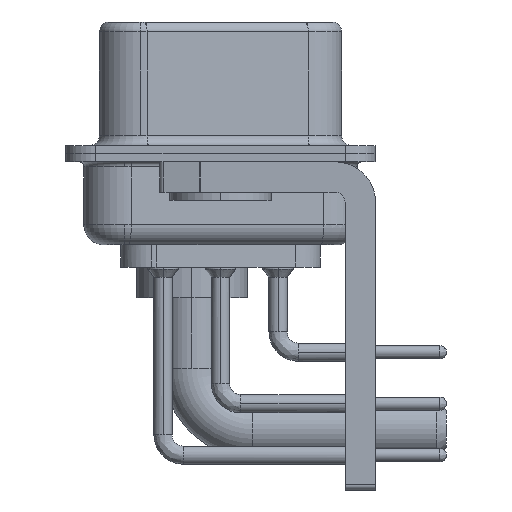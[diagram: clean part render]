
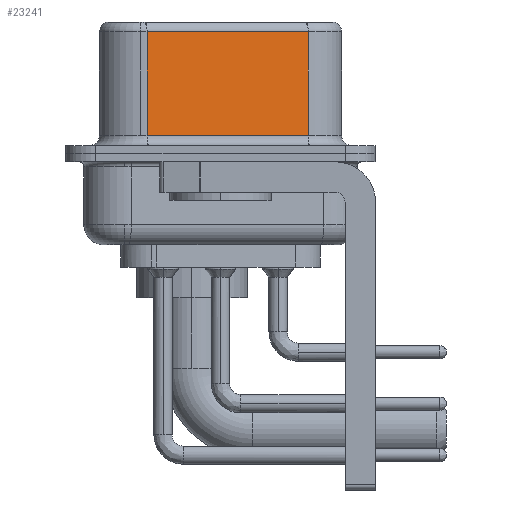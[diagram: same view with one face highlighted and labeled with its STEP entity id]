
A CAD part, left-side view. The second image highlights one B-rep face of the part: STEP entity #23241.
In plain terms, the highlighted planar face has unit normal (-0.985, -0.174, 0).
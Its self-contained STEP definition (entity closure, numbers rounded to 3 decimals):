
#31 = LINE ( 'NONE', #31865, #17573 ) ;
#104 = ORIENTED_EDGE ( 'NONE', *, *, #11338, .T. ) ;
#115 = CARTESIAN_POINT ( 'NONE',  ( 3.73, 3.628, 6.52 ) ) ;
#1654 = CARTESIAN_POINT ( 'NONE',  ( 5.132, -4.322, 6.02 ) ) ;
#2348 = DIRECTION ( 'NONE',  ( 0.985, 0.174, 0. ) ) ;
#4898 = AXIS2_PLACEMENT_3D ( 'NONE', #11787, #2348, #25856 ) ;
#5734 = EDGE_CURVE ( 'NONE', #5994, #14190, #31, .T. ) ;
#5755 = LINE ( 'NONE', #26366, #19918 ) ;
#5922 = DIRECTION ( 'NONE',  ( 0., 0., -1. ) ) ;
#5994 = VERTEX_POINT ( 'NONE', #1654 ) ;
#7140 = VERTEX_POINT ( 'NONE', #18262 ) ;
#9394 = CARTESIAN_POINT ( 'NONE',  ( 5.132, -4.322, 0.9 ) ) ;
#9592 = VECTOR ( 'NONE', #5922, 1000. ) ;
#10969 = DIRECTION ( 'NONE',  ( 0.174, -0.985, 0. ) ) ;
#11338 = EDGE_CURVE ( 'NONE', #7140, #14190, #5755, .T. ) ;
#11705 = LINE ( 'NONE', #115, #9592 ) ;
#11787 = CARTESIAN_POINT ( 'NONE',  ( 5.132, -4.322, 6.52 ) ) ;
#12642 = VECTOR ( 'NONE', #26289, 1000. ) ;
#12917 = EDGE_CURVE ( 'NONE', #5994, #19190, #13971, .T. ) ;
#13510 = CARTESIAN_POINT ( 'NONE',  ( 3.73, 3.628, 6.02 ) ) ;
#13971 = LINE ( 'NONE', #17236, #12642 ) ;
#14190 = VERTEX_POINT ( 'NONE', #9394 ) ;
#14327 = DIRECTION ( 'NONE',  ( 0., 0., -1. ) ) ;
#14500 = ORIENTED_EDGE ( 'NONE', *, *, #31309, .T. ) ;
#17236 = CARTESIAN_POINT ( 'NONE',  ( 5.132, -4.322, 6.02 ) ) ;
#17573 = VECTOR ( 'NONE', #14327, 1000. ) ;
#18262 = CARTESIAN_POINT ( 'NONE',  ( 3.73, 3.628, 0.9 ) ) ;
#19190 = VERTEX_POINT ( 'NONE', #13510 ) ;
#19918 = VECTOR ( 'NONE', #10969, 1000. ) ;
#23241 = ADVANCED_FACE ( 'NONE', ( #28754 ), #26051, .F. ) ;
#25856 = DIRECTION ( 'NONE',  ( -0.174, 0.985, 0. ) ) ;
#26051 = PLANE ( 'NONE',  #4898 ) ;
#26289 = DIRECTION ( 'NONE',  ( -0.174, 0.985, 0. ) ) ;
#26366 = CARTESIAN_POINT ( 'NONE',  ( 5.132, -4.322, 0.9 ) ) ;
#26873 = ORIENTED_EDGE ( 'NONE', *, *, #5734, .F. ) ;
#27369 = EDGE_LOOP ( 'NONE', ( #26873, #27593, #14500, #104 ) ) ;
#27593 = ORIENTED_EDGE ( 'NONE', *, *, #12917, .T. ) ;
#28754 = FACE_OUTER_BOUND ( 'NONE', #27369, .T. ) ;
#31309 = EDGE_CURVE ( 'NONE', #19190, #7140, #11705, .T. ) ;
#31865 = CARTESIAN_POINT ( 'NONE',  ( 5.132, -4.322, 6.52 ) ) ;
